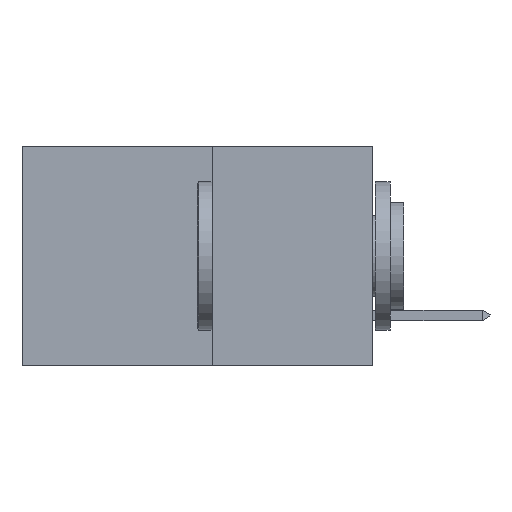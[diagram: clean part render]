
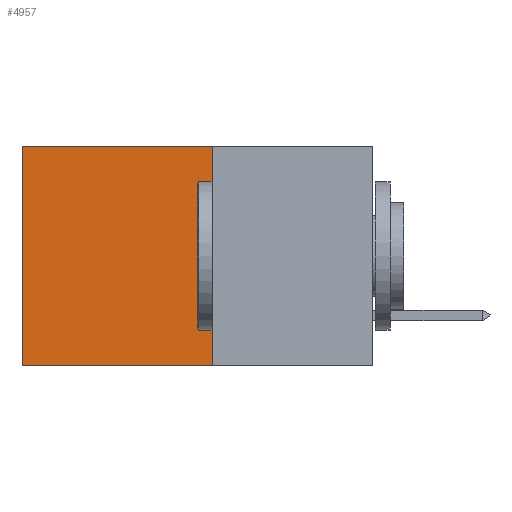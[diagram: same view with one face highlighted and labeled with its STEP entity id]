
A CAD part, left-side view. The second image highlights one B-rep face of the part: STEP entity #4957.
In plain terms, the highlighted planar face has unit normal (-1, 0, 0).
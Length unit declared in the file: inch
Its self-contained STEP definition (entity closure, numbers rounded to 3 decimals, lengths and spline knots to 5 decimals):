
#998 = CARTESIAN_POINT ( 'NONE',  ( 0.277, 0.27, -0.37 ) ) ;
#1028 = ORIENTED_EDGE ( 'NONE', *, *, #8747, .F. ) ;
#1655 = ORIENTED_EDGE ( 'NONE', *, *, #7364, .T. ) ;
#1933 = LINE ( 'NONE', #998, #3847 ) ;
#2059 = VECTOR ( 'NONE', #9258, 39.37008 ) ;
#2099 = CARTESIAN_POINT ( 'NONE',  ( 0.277, 0.27, 0. ) ) ;
#2154 = FACE_OUTER_BOUND ( 'NONE', #2594, .T. ) ;
#2594 = EDGE_LOOP ( 'NONE', ( #9706, #5764, #1028, #1655 ) ) ;
#2952 = DIRECTION ( 'NONE',  ( 0., 0., -1. ) ) ;
#3094 = CARTESIAN_POINT ( 'NONE',  ( 0.277, 0.59, -0.37 ) ) ;
#3499 = VERTEX_POINT ( 'NONE', #5843 ) ;
#3706 = CARTESIAN_POINT ( 'NONE',  ( 0.277, 0.27, -0.37 ) ) ;
#3778 = VECTOR ( 'NONE', #2952, 39.37008 ) ;
#3847 = VECTOR ( 'NONE', #4291, 39.37008 ) ;
#4291 = DIRECTION ( 'NONE',  ( 0., 1., 0. ) ) ;
#4558 = DIRECTION ( 'NONE',  ( 0., 1., 0. ) ) ;
#4686 = VERTEX_POINT ( 'NONE', #9547 ) ;
#4957 = ADVANCED_FACE ( 'NONE', ( #2154 ), #8001, .F. ) ;
#5764 = ORIENTED_EDGE ( 'NONE', *, *, #8543, .F. ) ;
#5843 = CARTESIAN_POINT ( 'NONE',  ( 0.277, 0.59, 0. ) ) ;
#5890 = EDGE_CURVE ( 'NONE', #3499, #4686, #6182, .T. ) ;
#5905 = VECTOR ( 'NONE', #4558, 39.37008 ) ;
#6182 = LINE ( 'NONE', #3094, #3778 ) ;
#6360 = LINE ( 'NONE', #3706, #2059 ) ;
#6368 = CARTESIAN_POINT ( 'NONE',  ( 0.277, 0.27, 0. ) ) ;
#6749 = AXIS2_PLACEMENT_3D ( 'NONE', #7989, #7984, #7982 ) ;
#6931 = CARTESIAN_POINT ( 'NONE',  ( 0.277, 0.27, -0.37 ) ) ;
#7364 = EDGE_CURVE ( 'NONE', #10292, #3499, #7991, .T. ) ;
#7982 = DIRECTION ( 'NONE',  ( 0., 0., -1. ) ) ;
#7984 = DIRECTION ( 'NONE',  ( 1., 0., 0. ) ) ;
#7989 = CARTESIAN_POINT ( 'NONE',  ( 0.277, 0.27, -0.37 ) ) ;
#7991 = LINE ( 'NONE', #2099, #5905 ) ;
#8001 = PLANE ( 'NONE',  #6749 ) ;
#8130 = VERTEX_POINT ( 'NONE', #6931 ) ;
#8543 = EDGE_CURVE ( 'NONE', #8130, #4686, #1933, .T. ) ;
#8747 = EDGE_CURVE ( 'NONE', #10292, #8130, #6360, .T. ) ;
#9258 = DIRECTION ( 'NONE',  ( 0., 0., -1. ) ) ;
#9547 = CARTESIAN_POINT ( 'NONE',  ( 0.277, 0.59, -0.37 ) ) ;
#9706 = ORIENTED_EDGE ( 'NONE', *, *, #5890, .T. ) ;
#10292 = VERTEX_POINT ( 'NONE', #6368 ) ;
